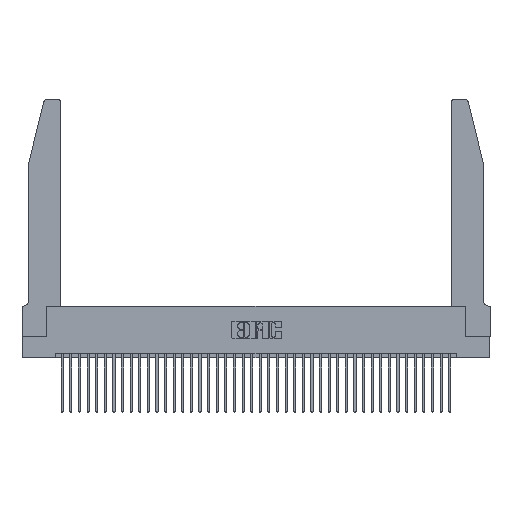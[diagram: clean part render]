
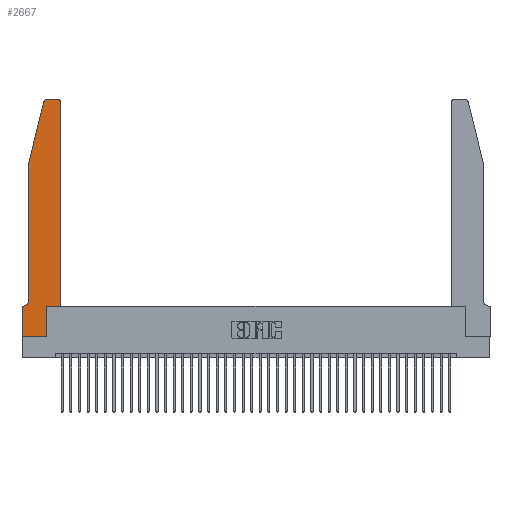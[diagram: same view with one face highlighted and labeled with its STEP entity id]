
A CAD part, top view. The second image highlights one B-rep face of the part: STEP entity #2667.
In plain terms, the highlighted planar face has unit normal (0, 0, 1).
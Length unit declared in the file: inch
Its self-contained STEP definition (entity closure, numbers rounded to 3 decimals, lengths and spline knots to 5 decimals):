
#192 = DIRECTION ( 'NONE',  ( 0., -1., 0. ) ) ;
#1037 = CARTESIAN_POINT ( 'NONE',  ( 0.0755, 0.35, 0.37 ) ) ;
#1158 = EDGE_CURVE ( 'NONE', #4575, #5200, #29939, .T. ) ;
#1825 = ORIENTED_EDGE ( 'NONE', *, *, #30928, .T. ) ;
#1893 = VERTEX_POINT ( 'NONE', #7467 ) ;
#2185 = CARTESIAN_POINT ( 'NONE',  ( 0., 0., 0.37 ) ) ;
#2261 = CARTESIAN_POINT ( 'NONE',  ( 0.0755, 2., 0.37 ) ) ;
#2372 = EDGE_CURVE ( 'NONE', #1893, #24960, #22226, .T. ) ;
#2667 = ADVANCED_FACE ( 'NONE', ( #18873 ), #35219, .T. ) ;
#3329 = VECTOR ( 'NONE', #14494, 39.37008 ) ;
#3408 = VERTEX_POINT ( 'NONE', #17563 ) ;
#3610 = CARTESIAN_POINT ( 'NONE',  ( 0.4505, 0.35, 0.37 ) ) ;
#3855 = ORIENTED_EDGE ( 'NONE', *, *, #23041, .T. ) ;
#4126 = LINE ( 'NONE', #5719, #36142 ) ;
#4193 = EDGE_CURVE ( 'NONE', #40206, #27152, #25471, .T. ) ;
#4372 = DIRECTION ( 'NONE',  ( -1., 0., 0. ) ) ;
#4575 = VERTEX_POINT ( 'NONE', #26249 ) ;
#4826 = CIRCLE ( 'NONE', #15689, 0.07 ) ;
#4952 = LINE ( 'NONE', #37447, #36907 ) ;
#5152 = DIRECTION ( 'NONE',  ( 0., 0., 1. ) ) ;
#5200 = VERTEX_POINT ( 'NONE', #30580 ) ;
#5557 = DIRECTION ( 'NONE',  ( 0., 0., -1. ) ) ;
#5719 = CARTESIAN_POINT ( 'NONE',  ( 0.2865, 0.35, 0.37 ) ) ;
#6582 = EDGE_CURVE ( 'NONE', #27152, #9239, #4126, .T. ) ;
#6892 = DIRECTION ( 'NONE',  ( 1., 0., 0. ) ) ;
#7410 = ORIENTED_EDGE ( 'NONE', *, *, #2372, .T. ) ;
#7467 = CARTESIAN_POINT ( 'NONE',  ( 0.25487, 2.72718, 0.37 ) ) ;
#9239 = VERTEX_POINT ( 'NONE', #18575 ) ;
#9947 = ORIENTED_EDGE ( 'NONE', *, *, #35712, .T. ) ;
#10060 = VECTOR ( 'NONE', #21084, 39.37008 ) ;
#10328 = EDGE_CURVE ( 'NONE', #29843, #3408, #4826, .T. ) ;
#11384 = CARTESIAN_POINT ( 'NONE',  ( 0.0755, 2., 0.37 ) ) ;
#11530 = CARTESIAN_POINT ( 'NONE',  ( 0.2605, 2.75, 0.37 ) ) ;
#11541 = VECTOR ( 'NONE', #4372, 39.37008 ) ;
#13378 = CIRCLE ( 'NONE', #13545, 0.03 ) ;
#13545 = AXIS2_PLACEMENT_3D ( 'NONE', #16269, #37650, #19386 ) ;
#13615 = CARTESIAN_POINT ( 'NONE',  ( 0.284, 2.75, 0.37 ) ) ;
#14494 = DIRECTION ( 'NONE',  ( 0., -1., 0. ) ) ;
#15248 = EDGE_LOOP ( 'NONE', ( #21061, #29168, #7410, #3855, #38754, #15317, #9947, #26338, #23974, #25871, #1825, #28742 ) ) ;
#15317 = ORIENTED_EDGE ( 'NONE', *, *, #27490, .T. ) ;
#15689 = AXIS2_PLACEMENT_3D ( 'NONE', #24214, #5557, #27260 ) ;
#16269 = CARTESIAN_POINT ( 'NONE',  ( 0.284, 2.72, 0.37 ) ) ;
#16284 = AXIS2_PLACEMENT_3D ( 'NONE', #23856, #5152, #26896 ) ;
#16544 = CARTESIAN_POINT ( 'NONE',  ( 0.0755, 0.42, 0.37 ) ) ;
#16925 = DIRECTION ( 'NONE',  ( 0., 0., 1. ) ) ;
#17563 = CARTESIAN_POINT ( 'NONE',  ( 0.0055, 0.35, 0.37 ) ) ;
#18575 = CARTESIAN_POINT ( 'NONE',  ( 0.2865, 0.35, 0.37 ) ) ;
#18873 = FACE_OUTER_BOUND ( 'NONE', #15248, .T. ) ;
#19225 = CARTESIAN_POINT ( 'NONE',  ( 0., 0., 0.37 ) ) ;
#19386 = DIRECTION ( 'NONE',  ( 1., 0., 0. ) ) ;
#19405 = VERTEX_POINT ( 'NONE', #13615 ) ;
#19438 = AXIS2_PLACEMENT_3D ( 'NONE', #29055, #16925, #38274 ) ;
#20903 = EDGE_CURVE ( 'NONE', #9239, #34074, #31185, .T. ) ;
#21061 = ORIENTED_EDGE ( 'NONE', *, *, #39861, .T. ) ;
#21084 = DIRECTION ( 'NONE',  ( 1., 0., 0. ) ) ;
#22226 = LINE ( 'NONE', #36964, #36552 ) ;
#22731 = EDGE_CURVE ( 'NONE', #19405, #1893, #13378, .T. ) ;
#22783 = CARTESIAN_POINT ( 'NONE',  ( 0.4505, 0.35, 0.37 ) ) ;
#23041 = EDGE_CURVE ( 'NONE', #24960, #29843, #28220, .T. ) ;
#23087 = VECTOR ( 'NONE', #6892, 39.37008 ) ;
#23617 = CARTESIAN_POINT ( 'NONE',  ( 0., 0.35, 0.37 ) ) ;
#23856 = CARTESIAN_POINT ( 'NONE',  ( 0.4205, 2.72, 0.37 ) ) ;
#23974 = ORIENTED_EDGE ( 'NONE', *, *, #6582, .T. ) ;
#24214 = CARTESIAN_POINT ( 'NONE',  ( 0.0055, 0.42, 0.37 ) ) ;
#24633 = DIRECTION ( 'NONE',  ( 0., 1., 0. ) ) ;
#24960 = VERTEX_POINT ( 'NONE', #2261 ) ;
#25283 = CARTESIAN_POINT ( 'NONE',  ( 0.4505, 0.35, 0.37 ) ) ;
#25471 = LINE ( 'NONE', #2185, #10060 ) ;
#25871 = ORIENTED_EDGE ( 'NONE', *, *, #20903, .T. ) ;
#26249 = CARTESIAN_POINT ( 'NONE',  ( 0.4505, 2.72, 0.37 ) ) ;
#26338 = ORIENTED_EDGE ( 'NONE', *, *, #4193, .T. ) ;
#26896 = DIRECTION ( 'NONE',  ( 1., 0., 0. ) ) ;
#27152 = VERTEX_POINT ( 'NONE', #33840 ) ;
#27260 = DIRECTION ( 'NONE',  ( -1., 0., 0. ) ) ;
#27490 = EDGE_CURVE ( 'NONE', #3408, #33654, #35045, .T. ) ;
#28220 = LINE ( 'NONE', #11384, #3329 ) ;
#28587 = VECTOR ( 'NONE', #39123, 39.37008 ) ;
#28742 = ORIENTED_EDGE ( 'NONE', *, *, #1158, .T. ) ;
#29055 = CARTESIAN_POINT ( 'NONE',  ( 0., 0.35, 0.37 ) ) ;
#29168 = ORIENTED_EDGE ( 'NONE', *, *, #22731, .T. ) ;
#29843 = VERTEX_POINT ( 'NONE', #16544 ) ;
#29939 = CIRCLE ( 'NONE', #16284, 0.03 ) ;
#30580 = CARTESIAN_POINT ( 'NONE',  ( 0.4205, 2.75, 0.37 ) ) ;
#30928 = EDGE_CURVE ( 'NONE', #34074, #4575, #31016, .T. ) ;
#31016 = LINE ( 'NONE', #25283, #37247 ) ;
#31185 = LINE ( 'NONE', #3610, #23087 ) ;
#33654 = VERTEX_POINT ( 'NONE', #23617 ) ;
#33840 = CARTESIAN_POINT ( 'NONE',  ( 0.2865, 0., 0.37 ) ) ;
#34074 = VERTEX_POINT ( 'NONE', #22783 ) ;
#35045 = LINE ( 'NONE', #1037, #11541 ) ;
#35219 = PLANE ( 'NONE',  #19438 ) ;
#35712 = EDGE_CURVE ( 'NONE', #33654, #40206, #4952, .T. ) ;
#36142 = VECTOR ( 'NONE', #24633, 39.37008 ) ;
#36552 = VECTOR ( 'NONE', #40018, 39.37008 ) ;
#36733 = LINE ( 'NONE', #11530, #28587 ) ;
#36907 = VECTOR ( 'NONE', #192, 39.37008 ) ;
#36964 = CARTESIAN_POINT ( 'NONE',  ( 0.0755, 2., 0.37 ) ) ;
#37247 = VECTOR ( 'NONE', #37436, 39.37008 ) ;
#37436 = DIRECTION ( 'NONE',  ( 0., 1., 0. ) ) ;
#37447 = CARTESIAN_POINT ( 'NONE',  ( 0., 0., 0.37 ) ) ;
#37650 = DIRECTION ( 'NONE',  ( 0., 0., 1. ) ) ;
#38274 = DIRECTION ( 'NONE',  ( 1., 0., 0. ) ) ;
#38754 = ORIENTED_EDGE ( 'NONE', *, *, #10328, .T. ) ;
#39123 = DIRECTION ( 'NONE',  ( -1., 0., 0. ) ) ;
#39861 = EDGE_CURVE ( 'NONE', #5200, #19405, #36733, .T. ) ;
#40018 = DIRECTION ( 'NONE',  ( -0.239, -0.971, 0. ) ) ;
#40206 = VERTEX_POINT ( 'NONE', #19225 ) ;
